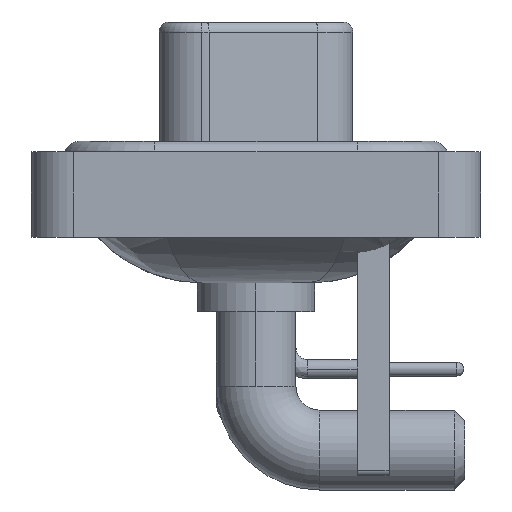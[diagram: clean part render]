
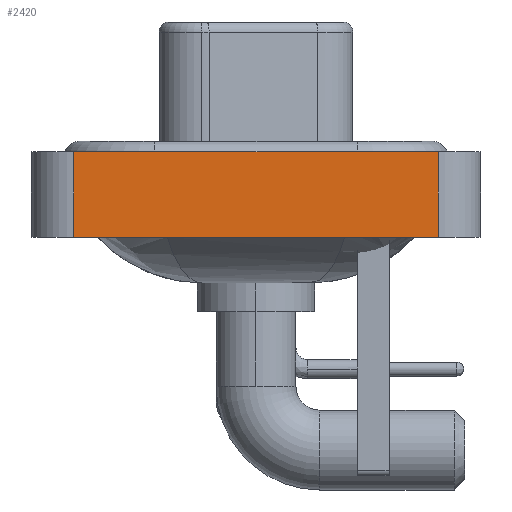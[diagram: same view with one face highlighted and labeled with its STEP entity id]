
A CAD part, left-side view. The second image highlights one B-rep face of the part: STEP entity #2420.
In plain terms, the highlighted planar face has unit normal (-1, 0, 0).
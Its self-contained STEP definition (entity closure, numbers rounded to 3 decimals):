
#858 = VERTEX_POINT ( 'NONE', #18982 ) ;
#1827 = VECTOR ( 'NONE', #11256, 1000. ) ;
#1906 = VERTEX_POINT ( 'NONE', #8796 ) ;
#2014 = LINE ( 'NONE', #3936, #23860 ) ;
#2420 = ADVANCED_FACE ( 'NONE', ( #6239 ), #26626, .T. ) ;
#2821 = VECTOR ( 'NONE', #16737, 1000. ) ;
#3373 = EDGE_LOOP ( 'NONE', ( #20472, #17824, #12774, #28903 ) ) ;
#3527 = CARTESIAN_POINT ( 'NONE',  ( -7.35, 8.55, -3.6 ) ) ;
#3936 = CARTESIAN_POINT ( 'NONE',  ( -7.35, -8.55, 0.4 ) ) ;
#4953 = AXIS2_PLACEMENT_3D ( 'NONE', #24134, #6546, #19535 ) ;
#5315 = LINE ( 'NONE', #3527, #28937 ) ;
#6239 = FACE_OUTER_BOUND ( 'NONE', #3373, .T. ) ;
#6546 = DIRECTION ( 'NONE',  ( -1., 0., 0. ) ) ;
#7735 = CARTESIAN_POINT ( 'NONE',  ( -7.35, -8.55, -3.6 ) ) ;
#8796 = CARTESIAN_POINT ( 'NONE',  ( -7.35, -8.55, -3.6 ) ) ;
#8869 = LINE ( 'NONE', #13603, #1827 ) ;
#10603 = DIRECTION ( 'NONE',  ( 0., -1., 0. ) ) ;
#11256 = DIRECTION ( 'NONE',  ( 0., 0., 1. ) ) ;
#12564 = DIRECTION ( 'NONE',  ( 0., 0., 1. ) ) ;
#12774 = ORIENTED_EDGE ( 'NONE', *, *, #26593, .F. ) ;
#12832 = CARTESIAN_POINT ( 'NONE',  ( -7.35, 8.55, 0.4 ) ) ;
#13603 = CARTESIAN_POINT ( 'NONE',  ( -7.35, -8.55, -3.6 ) ) ;
#14620 = EDGE_CURVE ( 'NONE', #23718, #1906, #21171, .T. ) ;
#15204 = CARTESIAN_POINT ( 'NONE',  ( -7.35, 8.55, -3.6 ) ) ;
#16737 = DIRECTION ( 'NONE',  ( 0., -1., 0. ) ) ;
#17824 = ORIENTED_EDGE ( 'NONE', *, *, #28411, .F. ) ;
#18982 = CARTESIAN_POINT ( 'NONE',  ( -7.35, -8.55, 0.4 ) ) ;
#19535 = DIRECTION ( 'NONE',  ( 0., 0., 1. ) ) ;
#20472 = ORIENTED_EDGE ( 'NONE', *, *, #23127, .T. ) ;
#21171 = LINE ( 'NONE', #7735, #2821 ) ;
#23127 = EDGE_CURVE ( 'NONE', #1906, #858, #8869, .T. ) ;
#23718 = VERTEX_POINT ( 'NONE', #15204 ) ;
#23860 = VECTOR ( 'NONE', #10603, 1000. ) ;
#24134 = CARTESIAN_POINT ( 'NONE',  ( -7.35, -8.55, -3.6 ) ) ;
#26593 = EDGE_CURVE ( 'NONE', #23718, #28397, #5315, .T. ) ;
#26626 = PLANE ( 'NONE',  #4953 ) ;
#28397 = VERTEX_POINT ( 'NONE', #12832 ) ;
#28411 = EDGE_CURVE ( 'NONE', #28397, #858, #2014, .T. ) ;
#28903 = ORIENTED_EDGE ( 'NONE', *, *, #14620, .T. ) ;
#28937 = VECTOR ( 'NONE', #12564, 1000. ) ;
